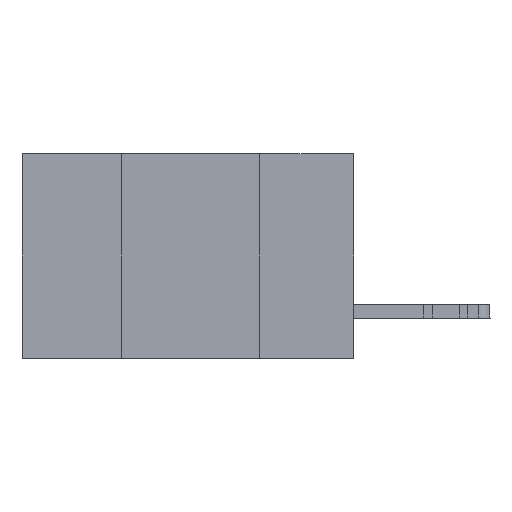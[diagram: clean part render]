
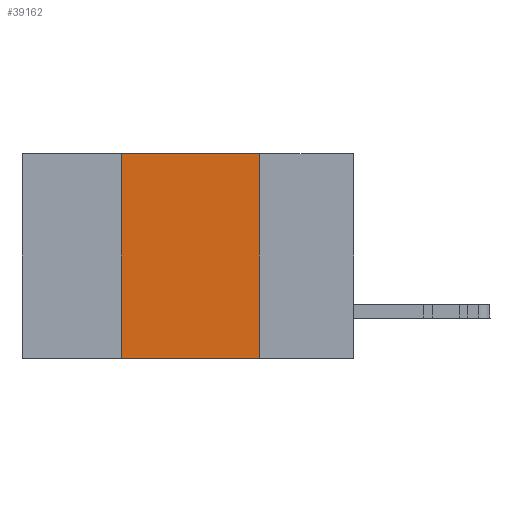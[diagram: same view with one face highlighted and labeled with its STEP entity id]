
A CAD part, left-side view. The second image highlights one B-rep face of the part: STEP entity #39162.
In plain terms, the highlighted planar face has unit normal (-1, 0, 0).
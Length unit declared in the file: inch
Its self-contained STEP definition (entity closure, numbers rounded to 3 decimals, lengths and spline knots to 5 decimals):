
#146 = CARTESIAN_POINT ( 'NONE',  ( 0., 0.42, 0. ) ) ;
#2143 = ORIENTED_EDGE ( 'NONE', *, *, #21598, .F. ) ;
#3042 = CARTESIAN_POINT ( 'NONE',  ( 0., 0.6, 0. ) ) ;
#3503 = ORIENTED_EDGE ( 'NONE', *, *, #36353, .F. ) ;
#4587 = CARTESIAN_POINT ( 'NONE',  ( 0., 0.6, -0.37 ) ) ;
#5365 = VERTEX_POINT ( 'NONE', #27079 ) ;
#6626 = VECTOR ( 'NONE', #8871, 39.37008 ) ;
#8871 = DIRECTION ( 'NONE',  ( 0., -1., 0. ) ) ;
#9463 = LINE ( 'NONE', #3042, #6626 ) ;
#9779 = DIRECTION ( 'NONE',  ( 1., 0., 0. ) ) ;
#12106 = VERTEX_POINT ( 'NONE', #16037 ) ;
#12627 = DIRECTION ( 'NONE',  ( 0., 0., -1. ) ) ;
#13018 = FACE_OUTER_BOUND ( 'NONE', #24647, .T. ) ;
#13214 = CARTESIAN_POINT ( 'NONE',  ( 0., 0.6, 0. ) ) ;
#13227 = EDGE_CURVE ( 'NONE', #5365, #17156, #18116, .T. ) ;
#14780 = CARTESIAN_POINT ( 'NONE',  ( 0., 0.17, 0. ) ) ;
#14885 = EDGE_CURVE ( 'NONE', #5365, #12106, #32170, .T. ) ;
#16037 = CARTESIAN_POINT ( 'NONE',  ( 0., 0.17, -0.37 ) ) ;
#17156 = VERTEX_POINT ( 'NONE', #146 ) ;
#17864 = CARTESIAN_POINT ( 'NONE',  ( 0., 0.17, 0. ) ) ;
#18116 = LINE ( 'NONE', #26563, #36145 ) ;
#21598 = EDGE_CURVE ( 'NONE', #17156, #30229, #9463, .T. ) ;
#22647 = ORIENTED_EDGE ( 'NONE', *, *, #14885, .T. ) ;
#22713 = VECTOR ( 'NONE', #28941, 39.37008 ) ;
#24647 = EDGE_LOOP ( 'NONE', ( #3503, #2143, #38079, #22647 ) ) ;
#25075 = AXIS2_PLACEMENT_3D ( 'NONE', #13214, #9779, #12627 ) ;
#26563 = CARTESIAN_POINT ( 'NONE',  ( 0., 0.42, 0. ) ) ;
#26916 = LINE ( 'NONE', #17864, #29392 ) ;
#27079 = CARTESIAN_POINT ( 'NONE',  ( 0., 0.42, -0.37 ) ) ;
#27888 = PLANE ( 'NONE',  #25075 ) ;
#28941 = DIRECTION ( 'NONE',  ( 0., -1., 0. ) ) ;
#29392 = VECTOR ( 'NONE', #39538, 39.37008 ) ;
#30229 = VERTEX_POINT ( 'NONE', #14780 ) ;
#30373 = DIRECTION ( 'NONE',  ( 0., 0., 1. ) ) ;
#32170 = LINE ( 'NONE', #4587, #22713 ) ;
#36145 = VECTOR ( 'NONE', #30373, 39.37008 ) ;
#36353 = EDGE_CURVE ( 'NONE', #30229, #12106, #26916, .T. ) ;
#38079 = ORIENTED_EDGE ( 'NONE', *, *, #13227, .F. ) ;
#39162 = ADVANCED_FACE ( 'NONE', ( #13018 ), #27888, .F. ) ;
#39538 = DIRECTION ( 'NONE',  ( 0., 0., -1. ) ) ;
